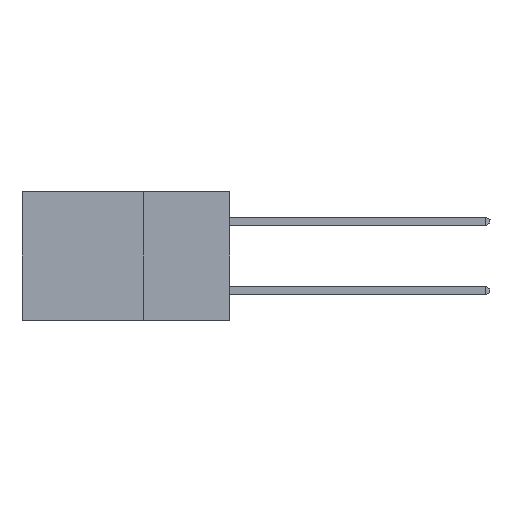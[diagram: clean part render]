
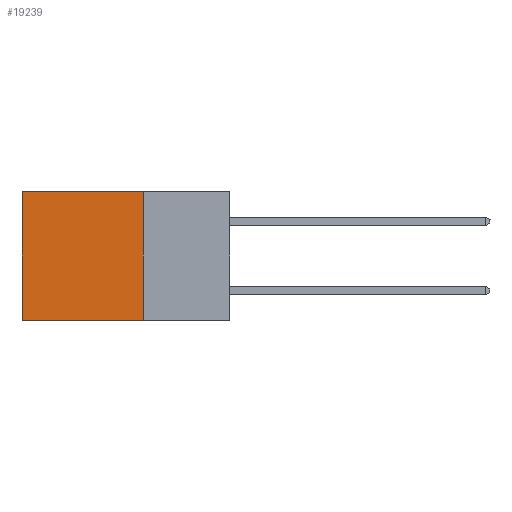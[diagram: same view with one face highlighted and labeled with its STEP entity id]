
A CAD part, left-side view. The second image highlights one B-rep face of the part: STEP entity #19239.
In plain terms, the highlighted planar face has unit normal (-1, 0, 0).
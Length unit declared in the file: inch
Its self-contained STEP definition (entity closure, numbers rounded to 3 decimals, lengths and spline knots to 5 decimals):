
#401 = EDGE_CURVE ( 'NONE', #24084, #4596, #14667, .T. ) ;
#708 = VECTOR ( 'NONE', #23073, 39.37008 ) ;
#941 = CARTESIAN_POINT ( 'NONE',  ( 0.298, 0.25, 0. ) ) ;
#1399 = DIRECTION ( 'NONE',  ( 0., 1., 0. ) ) ;
#1765 = PLANE ( 'NONE',  #12889 ) ;
#3021 = EDGE_LOOP ( 'NONE', ( #12301, #3920, #12260, #19516 ) ) ;
#3920 = ORIENTED_EDGE ( 'NONE', *, *, #13795, .F. ) ;
#4596 = VERTEX_POINT ( 'NONE', #8822 ) ;
#4996 = CARTESIAN_POINT ( 'NONE',  ( 0.298, 0.6, 0. ) ) ;
#5015 = EDGE_CURVE ( 'NONE', #19904, #24084, #18981, .T. ) ;
#6181 = LINE ( 'NONE', #6784, #708 ) ;
#6784 = CARTESIAN_POINT ( 'NONE',  ( 0.298, 0.25, 0. ) ) ;
#7054 = LINE ( 'NONE', #17648, #24779 ) ;
#7726 = DIRECTION ( 'NONE',  ( 1., 0., 0. ) ) ;
#8588 = CARTESIAN_POINT ( 'NONE',  ( 0.298, 0.25, 0. ) ) ;
#8822 = CARTESIAN_POINT ( 'NONE',  ( 0.298, 0.6, -0.37 ) ) ;
#9503 = VECTOR ( 'NONE', #25799, 39.37008 ) ;
#9777 = DIRECTION ( 'NONE',  ( 0., 1., 0. ) ) ;
#9890 = DIRECTION ( 'NONE',  ( 0., 0., -1. ) ) ;
#10357 = FACE_OUTER_BOUND ( 'NONE', #3021, .T. ) ;
#11711 = CARTESIAN_POINT ( 'NONE',  ( 0.298, 0.25, 0. ) ) ;
#11852 = EDGE_CURVE ( 'NONE', #19904, #19170, #6181, .T. ) ;
#12260 = ORIENTED_EDGE ( 'NONE', *, *, #11852, .F. ) ;
#12301 = ORIENTED_EDGE ( 'NONE', *, *, #401, .T. ) ;
#12889 = AXIS2_PLACEMENT_3D ( 'NONE', #11711, #7726, #9890 ) ;
#13677 = CARTESIAN_POINT ( 'NONE',  ( 0.298, 0.25, -0.37 ) ) ;
#13795 = EDGE_CURVE ( 'NONE', #19170, #4596, #7054, .T. ) ;
#14667 = LINE ( 'NONE', #4996, #9503 ) ;
#17648 = CARTESIAN_POINT ( 'NONE',  ( 0.298, 0.25, -0.37 ) ) ;
#18410 = CARTESIAN_POINT ( 'NONE',  ( 0.298, 0.6, 0. ) ) ;
#18981 = LINE ( 'NONE', #941, #21548 ) ;
#19170 = VERTEX_POINT ( 'NONE', #13677 ) ;
#19239 = ADVANCED_FACE ( 'NONE', ( #10357 ), #1765, .F. ) ;
#19516 = ORIENTED_EDGE ( 'NONE', *, *, #5015, .T. ) ;
#19904 = VERTEX_POINT ( 'NONE', #8588 ) ;
#21548 = VECTOR ( 'NONE', #9777, 39.37008 ) ;
#23073 = DIRECTION ( 'NONE',  ( 0., 0., -1. ) ) ;
#24084 = VERTEX_POINT ( 'NONE', #18410 ) ;
#24779 = VECTOR ( 'NONE', #1399, 39.37008 ) ;
#25799 = DIRECTION ( 'NONE',  ( 0., 0., -1. ) ) ;
